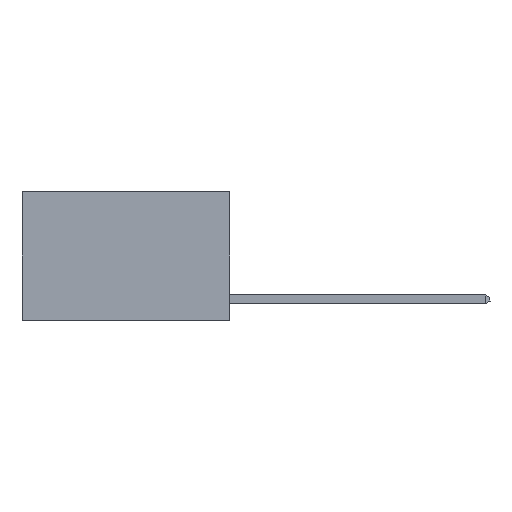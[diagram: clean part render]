
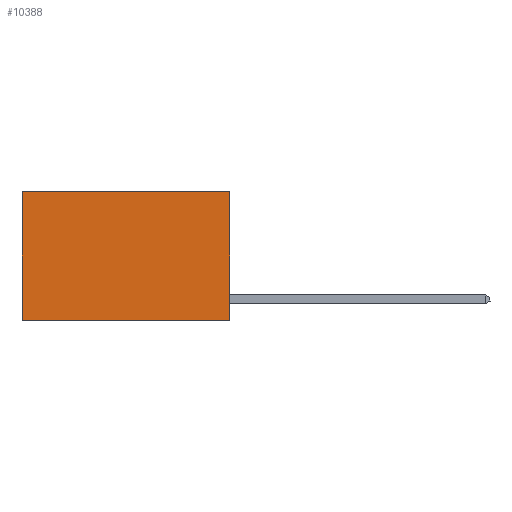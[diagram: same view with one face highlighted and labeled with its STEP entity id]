
A CAD part, left-side view. The second image highlights one B-rep face of the part: STEP entity #10388.
In plain terms, the highlighted planar face has unit normal (-1, 0, 0).
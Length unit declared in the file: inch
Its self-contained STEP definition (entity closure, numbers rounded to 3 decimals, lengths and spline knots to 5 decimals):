
#228 = CARTESIAN_POINT ( 'NONE',  ( 0.2625, 0., -0.37 ) ) ;
#1110 = CARTESIAN_POINT ( 'NONE',  ( 0.2625, 0., -0.37 ) ) ;
#2327 = CARTESIAN_POINT ( 'NONE',  ( 0.2625, 0., 0. ) ) ;
#2846 = LINE ( 'NONE', #1110, #9251 ) ;
#3409 = VERTEX_POINT ( 'NONE', #8382 ) ;
#3517 = DIRECTION ( 'NONE',  ( 0., 1., 0. ) ) ;
#3745 = EDGE_CURVE ( 'NONE', #3409, #14291, #10918, .T. ) ;
#4881 = CARTESIAN_POINT ( 'NONE',  ( 0.2625, 0.6, -0.37 ) ) ;
#4967 = VERTEX_POINT ( 'NONE', #22224 ) ;
#6006 = VECTOR ( 'NONE', #8739, 39.37008 ) ;
#6198 = EDGE_CURVE ( 'NONE', #14291, #10376, #2846, .T. ) ;
#7553 = ORIENTED_EDGE ( 'NONE', *, *, #6198, .F. ) ;
#8382 = CARTESIAN_POINT ( 'NONE',  ( 0.2625, 0., 0. ) ) ;
#8739 = DIRECTION ( 'NONE',  ( 0., 0., -1. ) ) ;
#8938 = DIRECTION ( 'NONE',  ( 0., 0., -1. ) ) ;
#9251 = VECTOR ( 'NONE', #3517, 39.37008 ) ;
#10376 = VERTEX_POINT ( 'NONE', #4881 ) ;
#10388 = ADVANCED_FACE ( 'NONE', ( #16795 ), #16602, .F. ) ;
#10490 = VECTOR ( 'NONE', #8938, 39.37008 ) ;
#10918 = LINE ( 'NONE', #12647, #6006 ) ;
#11866 = ORIENTED_EDGE ( 'NONE', *, *, #3745, .F. ) ;
#12647 = CARTESIAN_POINT ( 'NONE',  ( 0.2625, 0., 0. ) ) ;
#12830 = EDGE_CURVE ( 'NONE', #4967, #10376, #20896, .T. ) ;
#13067 = EDGE_LOOP ( 'NONE', ( #21940, #7553, #11866, #15769 ) ) ;
#14145 = DIRECTION ( 'NONE',  ( 0., 1., 0. ) ) ;
#14163 = LINE ( 'NONE', #2327, #20565 ) ;
#14291 = VERTEX_POINT ( 'NONE', #228 ) ;
#14854 = AXIS2_PLACEMENT_3D ( 'NONE', #22060, #22155, #24202 ) ;
#15769 = ORIENTED_EDGE ( 'NONE', *, *, #23666, .T. ) ;
#16602 = PLANE ( 'NONE',  #14854 ) ;
#16795 = FACE_OUTER_BOUND ( 'NONE', #13067, .T. ) ;
#18597 = CARTESIAN_POINT ( 'NONE',  ( 0.2625, 0.6, 0. ) ) ;
#20565 = VECTOR ( 'NONE', #14145, 39.37008 ) ;
#20896 = LINE ( 'NONE', #18597, #10490 ) ;
#21940 = ORIENTED_EDGE ( 'NONE', *, *, #12830, .T. ) ;
#22060 = CARTESIAN_POINT ( 'NONE',  ( 0.2625, 0., 0. ) ) ;
#22155 = DIRECTION ( 'NONE',  ( 1., 0., 0. ) ) ;
#22224 = CARTESIAN_POINT ( 'NONE',  ( 0.2625, 0.6, 0. ) ) ;
#23666 = EDGE_CURVE ( 'NONE', #3409, #4967, #14163, .T. ) ;
#24202 = DIRECTION ( 'NONE',  ( 0., 0., -1. ) ) ;
